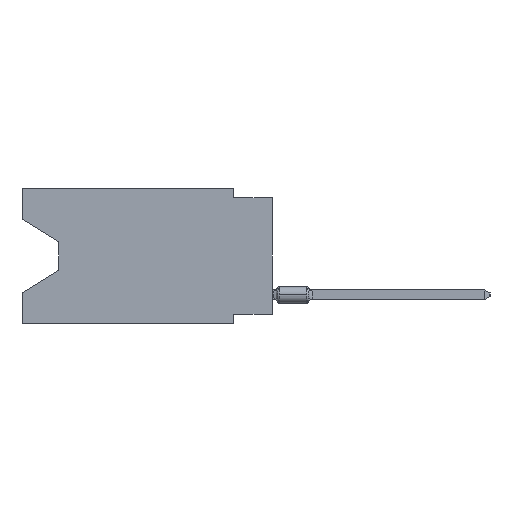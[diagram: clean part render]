
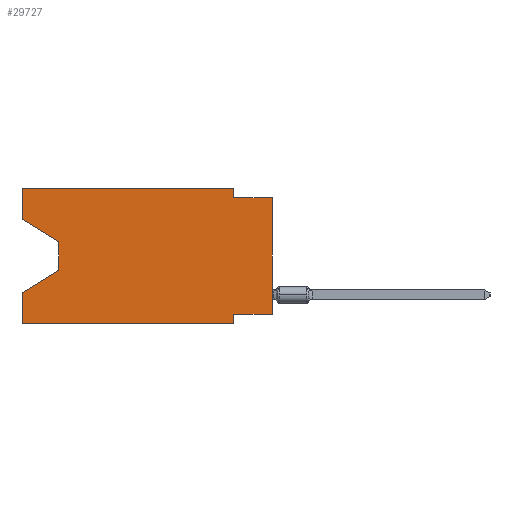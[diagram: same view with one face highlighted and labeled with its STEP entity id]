
A CAD part, left-side view. The second image highlights one B-rep face of the part: STEP entity #29727.
In plain terms, the highlighted planar face has unit normal (-1, 0, 0).
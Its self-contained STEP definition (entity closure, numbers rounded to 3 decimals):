
#428 = EDGE_CURVE ( 'NONE', #41778, #18246, #7808, .T. ) ;
#473 = CARTESIAN_POINT ( 'NONE',  ( 0., 0., -8.255 ) ) ;
#1295 = VECTOR ( 'NONE', #48240, 1000. ) ;
#1453 = CARTESIAN_POINT ( 'NONE',  ( 0., 0., -8.255 ) ) ;
#1842 = VECTOR ( 'NONE', #50483, 1000. ) ;
#2595 = VECTOR ( 'NONE', #2734, 1000. ) ;
#2734 = DIRECTION ( 'NONE',  ( 0., -0.855, -0.519 ) ) ;
#3270 = CARTESIAN_POINT ( 'NONE',  ( 0., 16.383, -8.89 ) ) ;
#3689 = ORIENTED_EDGE ( 'NONE', *, *, #27674, .F. ) ;
#4123 = FACE_OUTER_BOUND ( 'NONE', #23367, .T. ) ;
#4829 = VERTEX_POINT ( 'NONE', #49161 ) ;
#4958 = LINE ( 'NONE', #21495, #18860 ) ;
#5090 = AXIS2_PLACEMENT_3D ( 'NONE', #46645, #26541, #22190 ) ;
#5141 = DIRECTION ( 'NONE',  ( 0., 0.855, -0.519 ) ) ;
#5304 = LINE ( 'NONE', #50661, #46959 ) ;
#5334 = CARTESIAN_POINT ( 'NONE',  ( 0., 2.54, -8.89 ) ) ;
#5742 = EDGE_CURVE ( 'NONE', #18246, #32953, #17972, .T. ) ;
#7498 = VECTOR ( 'NONE', #51749, 1000. ) ;
#7808 = LINE ( 'NONE', #40117, #41983 ) ;
#8054 = CARTESIAN_POINT ( 'NONE',  ( 0., 16.383, 0. ) ) ;
#9124 = ORIENTED_EDGE ( 'NONE', *, *, #26429, .T. ) ;
#9224 = VERTEX_POINT ( 'NONE', #473 ) ;
#9318 = EDGE_CURVE ( 'NONE', #13627, #41778, #51213, .T. ) ;
#9538 = DIRECTION ( 'NONE',  ( 0., -1., 0. ) ) ;
#10777 = CARTESIAN_POINT ( 'NONE',  ( 0., 16.383, 0. ) ) ;
#11103 = CARTESIAN_POINT ( 'NONE',  ( 0., 16.383, -2.038 ) ) ;
#11425 = ORIENTED_EDGE ( 'NONE', *, *, #53599, .T. ) ;
#12461 = EDGE_CURVE ( 'NONE', #14686, #13627, #47971, .T. ) ;
#13273 = LINE ( 'NONE', #42325, #46603 ) ;
#13464 = LINE ( 'NONE', #5334, #7498 ) ;
#13627 = VERTEX_POINT ( 'NONE', #8054 ) ;
#14267 = DIRECTION ( 'NONE',  ( 0., -1., 0. ) ) ;
#14686 = VERTEX_POINT ( 'NONE', #11103 ) ;
#16622 = DIRECTION ( 'NONE',  ( 0., 0., 1. ) ) ;
#17158 = LINE ( 'NONE', #41881, #37997 ) ;
#17607 = CARTESIAN_POINT ( 'NONE',  ( 0., 13.97, -3.505 ) ) ;
#17972 = LINE ( 'NONE', #34540, #19085 ) ;
#18246 = VERTEX_POINT ( 'NONE', #37822 ) ;
#18860 = VECTOR ( 'NONE', #9538, 1000. ) ;
#19085 = VECTOR ( 'NONE', #33750, 1000. ) ;
#19479 = DIRECTION ( 'NONE',  ( 0., 0., -1. ) ) ;
#21495 = CARTESIAN_POINT ( 'NONE',  ( 0., 16.383, -8.89 ) ) ;
#21650 = CARTESIAN_POINT ( 'NONE',  ( 0., 16.383, -6.852 ) ) ;
#21670 = EDGE_CURVE ( 'NONE', #9224, #4829, #22076, .T. ) ;
#22076 = LINE ( 'NONE', #1453, #22109 ) ;
#22109 = VECTOR ( 'NONE', #38371, 1000. ) ;
#22190 = DIRECTION ( 'NONE',  ( 0., 0., -1. ) ) ;
#22465 = ORIENTED_EDGE ( 'NONE', *, *, #21670, .F. ) ;
#23367 = EDGE_LOOP ( 'NONE', ( #11425, #45836, #9124, #3689, #37202, #33382, #22465, #49116, #46025, #25324, #32952, #45358 ) ) ;
#23785 = CARTESIAN_POINT ( 'NONE',  ( 0., 2.54, 0. ) ) ;
#25324 = ORIENTED_EDGE ( 'NONE', *, *, #428, .F. ) ;
#25674 = EDGE_CURVE ( 'NONE', #4829, #35450, #13464, .T. ) ;
#26429 = EDGE_CURVE ( 'NONE', #47369, #47187, #13273, .T. ) ;
#26541 = DIRECTION ( 'NONE',  ( 1., 0., 0. ) ) ;
#27674 = EDGE_CURVE ( 'NONE', #32293, #47187, #17158, .T. ) ;
#29202 = DIRECTION ( 'NONE',  ( 0., 0., 1. ) ) ;
#29727 = ADVANCED_FACE ( 'NONE', ( #4123 ), #42308, .F. ) ;
#30835 = CARTESIAN_POINT ( 'NONE',  ( 0., 16.383, 0. ) ) ;
#31515 = CARTESIAN_POINT ( 'NONE',  ( 0., 16.383, -2.038 ) ) ;
#32293 = VERTEX_POINT ( 'NONE', #3270 ) ;
#32953 = VERTEX_POINT ( 'NONE', #45181 ) ;
#32952 = ORIENTED_EDGE ( 'NONE', *, *, #9318, .F. ) ;
#33382 = ORIENTED_EDGE ( 'NONE', *, *, #25674, .F. ) ;
#33750 = DIRECTION ( 'NONE',  ( 0., -1., 0. ) ) ;
#34540 = CARTESIAN_POINT ( 'NONE',  ( 0., 0., -0.635 ) ) ;
#35310 = LINE ( 'NONE', #31515, #2595 ) ;
#35450 = VERTEX_POINT ( 'NONE', #40290 ) ;
#35951 = CARTESIAN_POINT ( 'NONE',  ( 0., 13.97, -3.505 ) ) ;
#37202 = ORIENTED_EDGE ( 'NONE', *, *, #51027, .T. ) ;
#37822 = CARTESIAN_POINT ( 'NONE',  ( 0., 2.54, -0.635 ) ) ;
#37997 = VECTOR ( 'NONE', #16622, 1000. ) ;
#38371 = DIRECTION ( 'NONE',  ( 0., 1., 0. ) ) ;
#39775 = EDGE_CURVE ( 'NONE', #43430, #47369, #43853, .T. ) ;
#40117 = CARTESIAN_POINT ( 'NONE',  ( 0., 2.54, 0. ) ) ;
#40290 = CARTESIAN_POINT ( 'NONE',  ( 0., 2.54, -8.89 ) ) ;
#41778 = VERTEX_POINT ( 'NONE', #23785 ) ;
#41881 = CARTESIAN_POINT ( 'NONE',  ( 0., 16.383, 0. ) ) ;
#41983 = VECTOR ( 'NONE', #19479, 1000. ) ;
#42308 = PLANE ( 'NONE',  #5090 ) ;
#42325 = CARTESIAN_POINT ( 'NONE',  ( 0., 13.97, -5.385 ) ) ;
#43430 = VERTEX_POINT ( 'NONE', #35951 ) ;
#43853 = LINE ( 'NONE', #17607, #1842 ) ;
#44967 = CARTESIAN_POINT ( 'NONE',  ( 0., 13.97, -5.385 ) ) ;
#45181 = CARTESIAN_POINT ( 'NONE',  ( 0., 0., -0.635 ) ) ;
#45358 = ORIENTED_EDGE ( 'NONE', *, *, #12461, .F. ) ;
#45763 = EDGE_CURVE ( 'NONE', #9224, #32953, #5304, .T. ) ;
#45836 = ORIENTED_EDGE ( 'NONE', *, *, #39775, .T. ) ;
#46025 = ORIENTED_EDGE ( 'NONE', *, *, #5742, .F. ) ;
#46603 = VECTOR ( 'NONE', #5141, 1000. ) ;
#46645 = CARTESIAN_POINT ( 'NONE',  ( 0., 16.383, 0. ) ) ;
#46959 = VECTOR ( 'NONE', #29202, 1000. ) ;
#47187 = VERTEX_POINT ( 'NONE', #21650 ) ;
#47369 = VERTEX_POINT ( 'NONE', #44967 ) ;
#47971 = LINE ( 'NONE', #10777, #1295 ) ;
#48240 = DIRECTION ( 'NONE',  ( 0., 0., 1. ) ) ;
#49116 = ORIENTED_EDGE ( 'NONE', *, *, #45763, .T. ) ;
#49161 = CARTESIAN_POINT ( 'NONE',  ( 0., 2.54, -8.255 ) ) ;
#49782 = VECTOR ( 'NONE', #14267, 1000. ) ;
#50483 = DIRECTION ( 'NONE',  ( 0., 0., -1. ) ) ;
#50661 = CARTESIAN_POINT ( 'NONE',  ( 0., 0., 0. ) ) ;
#51027 = EDGE_CURVE ( 'NONE', #32293, #35450, #4958, .T. ) ;
#51213 = LINE ( 'NONE', #30835, #49782 ) ;
#51749 = DIRECTION ( 'NONE',  ( 0., 0., -1. ) ) ;
#53599 = EDGE_CURVE ( 'NONE', #14686, #43430, #35310, .T. ) ;
